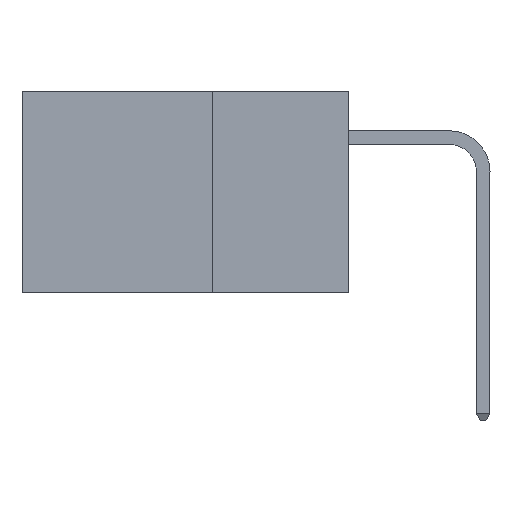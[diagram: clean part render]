
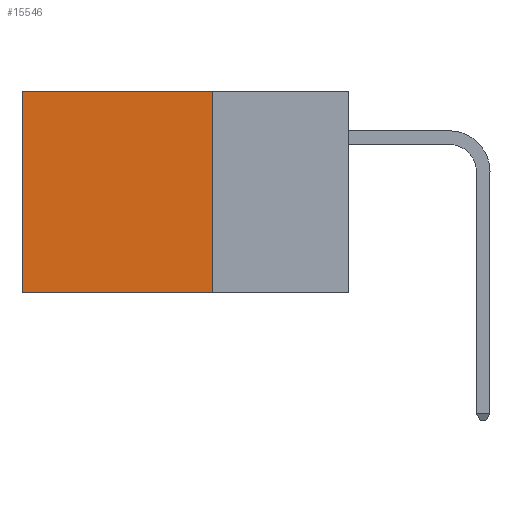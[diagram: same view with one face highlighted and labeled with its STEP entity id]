
A CAD part, left-side view. The second image highlights one B-rep face of the part: STEP entity #15546.
In plain terms, the highlighted planar face has unit normal (-1, 0, 0).
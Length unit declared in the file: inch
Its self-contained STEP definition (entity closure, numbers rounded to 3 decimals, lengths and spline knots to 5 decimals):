
#2235 = VECTOR ( 'NONE', #19923, 39.37008 ) ;
#2289 = LINE ( 'NONE', #14311, #12227 ) ;
#3166 = DIRECTION ( 'NONE',  ( 0., 0., -1. ) ) ;
#4645 = ORIENTED_EDGE ( 'NONE', *, *, #19305, .F. ) ;
#4804 = CARTESIAN_POINT ( 'NONE',  ( 0.2875, 0.25, 0. ) ) ;
#5247 = CARTESIAN_POINT ( 'NONE',  ( 0.2875, 0.25, 0. ) ) ;
#5766 = DIRECTION ( 'NONE',  ( 1., 0., 0. ) ) ;
#6905 = CARTESIAN_POINT ( 'NONE',  ( 0.2875, 0.25, 0. ) ) ;
#8611 = EDGE_CURVE ( 'NONE', #11210, #9329, #20633, .T. ) ;
#9329 = VERTEX_POINT ( 'NONE', #10493 ) ;
#9344 = CARTESIAN_POINT ( 'NONE',  ( 0.2875, 0.25, -0.37 ) ) ;
#9504 = CARTESIAN_POINT ( 'NONE',  ( 0.2875, 0.25, -0.37 ) ) ;
#9598 = ORIENTED_EDGE ( 'NONE', *, *, #8611, .T. ) ;
#10278 = DIRECTION ( 'NONE',  ( 0., 1., 0. ) ) ;
#10493 = CARTESIAN_POINT ( 'NONE',  ( 0.2875, 0.6, 0. ) ) ;
#11210 = VERTEX_POINT ( 'NONE', #5247 ) ;
#11728 = ORIENTED_EDGE ( 'NONE', *, *, #13635, .F. ) ;
#11896 = LINE ( 'NONE', #9344, #22416 ) ;
#12227 = VECTOR ( 'NONE', #3166, 39.37008 ) ;
#13635 = EDGE_CURVE ( 'NONE', #17287, #19274, #11896, .T. ) ;
#14311 = CARTESIAN_POINT ( 'NONE',  ( 0.2875, 0.6, 0. ) ) ;
#15244 = FACE_OUTER_BOUND ( 'NONE', #21993, .T. ) ;
#15546 = ADVANCED_FACE ( 'NONE', ( #15244 ), #24226, .F. ) ;
#16227 = VECTOR ( 'NONE', #10278, 39.37008 ) ;
#16879 = CARTESIAN_POINT ( 'NONE',  ( 0.2875, 0.25, 0. ) ) ;
#17287 = VERTEX_POINT ( 'NONE', #9504 ) ;
#18758 = DIRECTION ( 'NONE',  ( 0., 0., -1. ) ) ;
#19274 = VERTEX_POINT ( 'NONE', #21647 ) ;
#19305 = EDGE_CURVE ( 'NONE', #11210, #17287, #22663, .T. ) ;
#19733 = ORIENTED_EDGE ( 'NONE', *, *, #22723, .T. ) ;
#19923 = DIRECTION ( 'NONE',  ( 0., 0., -1. ) ) ;
#20633 = LINE ( 'NONE', #4804, #16227 ) ;
#21647 = CARTESIAN_POINT ( 'NONE',  ( 0.2875, 0.6, -0.37 ) ) ;
#21993 = EDGE_LOOP ( 'NONE', ( #19733, #11728, #4645, #9598 ) ) ;
#22105 = AXIS2_PLACEMENT_3D ( 'NONE', #16879, #5766, #18758 ) ;
#22405 = DIRECTION ( 'NONE',  ( 0., 1., 0. ) ) ;
#22416 = VECTOR ( 'NONE', #22405, 39.37008 ) ;
#22663 = LINE ( 'NONE', #6905, #2235 ) ;
#22723 = EDGE_CURVE ( 'NONE', #9329, #19274, #2289, .T. ) ;
#24226 = PLANE ( 'NONE',  #22105 ) ;
